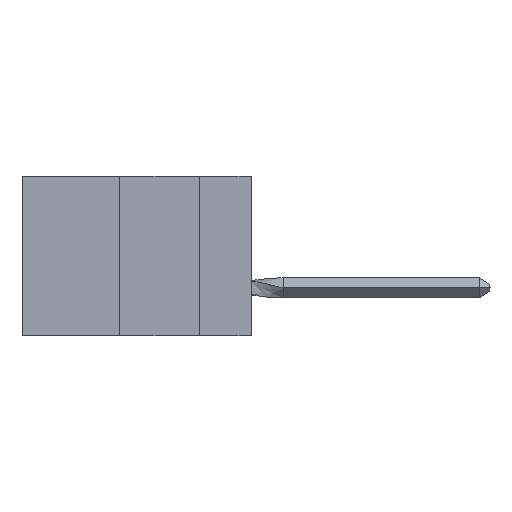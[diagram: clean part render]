
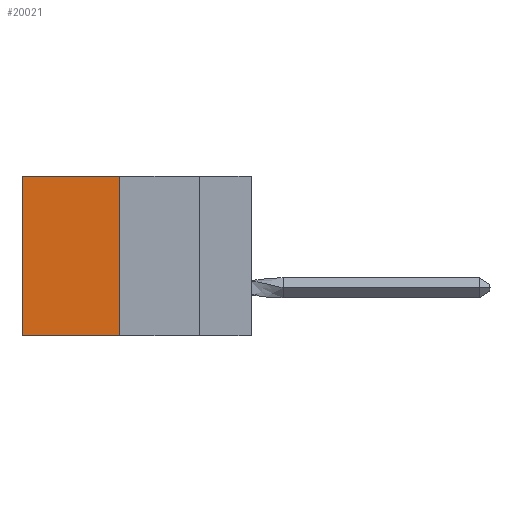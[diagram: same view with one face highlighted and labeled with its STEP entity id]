
A CAD part, left-side view. The second image highlights one B-rep face of the part: STEP entity #20021.
In plain terms, the highlighted planar face has unit normal (-1, 0, 0).
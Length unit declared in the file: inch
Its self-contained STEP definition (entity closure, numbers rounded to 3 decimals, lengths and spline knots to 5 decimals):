
#229 = VECTOR ( 'NONE', #10584, 39.37008 ) ;
#774 = ORIENTED_EDGE ( 'NONE', *, *, #31731, .T. ) ;
#1060 = ORIENTED_EDGE ( 'NONE', *, *, #24455, .T. ) ;
#1949 = DIRECTION ( 'NONE',  ( 1., 0., 0. ) ) ;
#1984 = DIRECTION ( 'NONE',  ( 0., 1., 0. ) ) ;
#3760 = ORIENTED_EDGE ( 'NONE', *, *, #26212, .F. ) ;
#4774 = EDGE_LOOP ( 'NONE', ( #1060, #7926, #3760, #774 ) ) ;
#4863 = CARTESIAN_POINT ( 'NONE',  ( 0.305, 0.413, -0.5 ) ) ;
#6375 = CARTESIAN_POINT ( 'NONE',  ( 0.305, 0.413, 0. ) ) ;
#7317 = CARTESIAN_POINT ( 'NONE',  ( 0.305, 0.72, 0. ) ) ;
#7815 = VECTOR ( 'NONE', #14680, 39.37008 ) ;
#7926 = ORIENTED_EDGE ( 'NONE', *, *, #24174, .F. ) ;
#8444 = DIRECTION ( 'NONE',  ( 0., 0., -1. ) ) ;
#10584 = DIRECTION ( 'NONE',  ( 0., 0., -1. ) ) ;
#11159 = LINE ( 'NONE', #4863, #24795 ) ;
#11792 = CARTESIAN_POINT ( 'NONE',  ( 0.305, 0.72, -0.5 ) ) ;
#14175 = FACE_OUTER_BOUND ( 'NONE', #4774, .T. ) ;
#14680 = DIRECTION ( 'NONE',  ( 0., 1., 0. ) ) ;
#15586 = CARTESIAN_POINT ( 'NONE',  ( 0.305, 0.413, -0.5 ) ) ;
#17932 = VERTEX_POINT ( 'NONE', #7317 ) ;
#18548 = VECTOR ( 'NONE', #8444, 39.37008 ) ;
#18947 = CARTESIAN_POINT ( 'NONE',  ( 0.305, 0.413, 0. ) ) ;
#20021 = ADVANCED_FACE ( 'NONE', ( #14175 ), #27220, .F. ) ;
#21040 = LINE ( 'NONE', #21596, #18548 ) ;
#21224 = AXIS2_PLACEMENT_3D ( 'NONE', #22730, #1949, #33515 ) ;
#21303 = LINE ( 'NONE', #21307, #229 ) ;
#21307 = CARTESIAN_POINT ( 'NONE',  ( 0.305, 0.413, -0.5 ) ) ;
#21596 = CARTESIAN_POINT ( 'NONE',  ( 0.305, 0.72, -0.5 ) ) ;
#22135 = VERTEX_POINT ( 'NONE', #11792 ) ;
#22730 = CARTESIAN_POINT ( 'NONE',  ( 0.305, 0.413, -0.5 ) ) ;
#24174 = EDGE_CURVE ( 'NONE', #28803, #22135, #11159, .T. ) ;
#24455 = EDGE_CURVE ( 'NONE', #17932, #22135, #21040, .T. ) ;
#24795 = VECTOR ( 'NONE', #1984, 39.37008 ) ;
#26212 = EDGE_CURVE ( 'NONE', #30177, #28803, #21303, .T. ) ;
#27220 = PLANE ( 'NONE',  #21224 ) ;
#28376 = LINE ( 'NONE', #6375, #7815 ) ;
#28803 = VERTEX_POINT ( 'NONE', #15586 ) ;
#30177 = VERTEX_POINT ( 'NONE', #18947 ) ;
#31731 = EDGE_CURVE ( 'NONE', #30177, #17932, #28376, .T. ) ;
#33515 = DIRECTION ( 'NONE',  ( 0., 0., -1. ) ) ;
